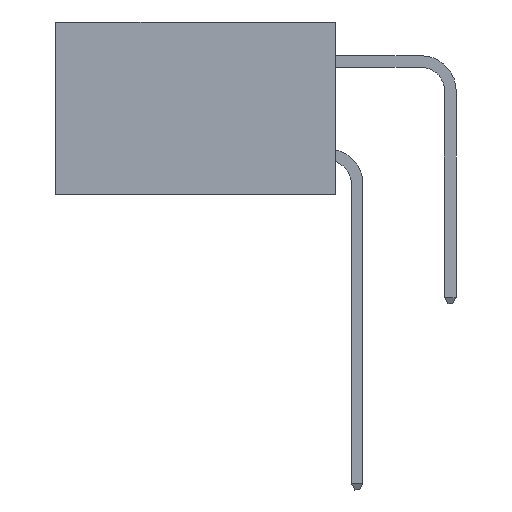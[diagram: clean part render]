
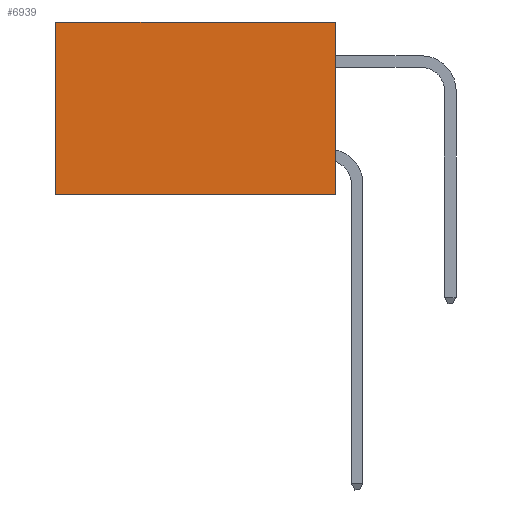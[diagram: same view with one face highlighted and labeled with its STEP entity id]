
A CAD part, left-side view. The second image highlights one B-rep face of the part: STEP entity #6939.
In plain terms, the highlighted planar face has unit normal (-1, 0, 0).
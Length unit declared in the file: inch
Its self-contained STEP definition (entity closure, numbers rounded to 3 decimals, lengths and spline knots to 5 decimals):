
#142 = CARTESIAN_POINT ( 'NONE',  ( 0.2875, 0.6, -0.37 ) ) ;
#578 = CARTESIAN_POINT ( 'NONE',  ( 0.2875, 0., -0.37 ) ) ;
#702 = CARTESIAN_POINT ( 'NONE',  ( 0.2875, 0., 0. ) ) ;
#854 = EDGE_CURVE ( 'NONE', #2070, #1374, #1759, .T. ) ;
#917 = LINE ( 'NONE', #3021, #9182 ) ;
#927 = CARTESIAN_POINT ( 'NONE',  ( 0.2875, 0.6, 0. ) ) ;
#1374 = VERTEX_POINT ( 'NONE', #142 ) ;
#1759 = LINE ( 'NONE', #578, #9862 ) ;
#1802 = DIRECTION ( 'NONE',  ( 0., 0., -1. ) ) ;
#2035 = AXIS2_PLACEMENT_3D ( 'NONE', #702, #8755, #4003 ) ;
#2070 = VERTEX_POINT ( 'NONE', #10262 ) ;
#2355 = VERTEX_POINT ( 'NONE', #4078 ) ;
#3021 = CARTESIAN_POINT ( 'NONE',  ( 0.2875, 0., 0. ) ) ;
#3191 = PLANE ( 'NONE',  #2035 ) ;
#3988 = VECTOR ( 'NONE', #9261, 39.37008 ) ;
#4003 = DIRECTION ( 'NONE',  ( 0., 0., -1. ) ) ;
#4078 = CARTESIAN_POINT ( 'NONE',  ( 0.2875, 0.6, 0. ) ) ;
#4181 = ORIENTED_EDGE ( 'NONE', *, *, #7413, .F. ) ;
#4833 = DIRECTION ( 'NONE',  ( 0., 1., 0. ) ) ;
#5002 = CARTESIAN_POINT ( 'NONE',  ( 0.2875, 0., 0. ) ) ;
#5904 = ORIENTED_EDGE ( 'NONE', *, *, #854, .F. ) ;
#6418 = LINE ( 'NONE', #927, #10190 ) ;
#6447 = EDGE_CURVE ( 'NONE', #2355, #1374, #6418, .T. ) ;
#6832 = EDGE_CURVE ( 'NONE', #7078, #2355, #917, .T. ) ;
#6939 = ADVANCED_FACE ( 'NONE', ( #8247 ), #3191, .F. ) ;
#7078 = VERTEX_POINT ( 'NONE', #5002 ) ;
#7413 = EDGE_CURVE ( 'NONE', #7078, #2070, #10174, .T. ) ;
#7451 = ORIENTED_EDGE ( 'NONE', *, *, #6832, .T. ) ;
#7495 = EDGE_LOOP ( 'NONE', ( #8118, #5904, #4181, #7451 ) ) ;
#7855 = DIRECTION ( 'NONE',  ( 0., 1., 0. ) ) ;
#8118 = ORIENTED_EDGE ( 'NONE', *, *, #6447, .T. ) ;
#8247 = FACE_OUTER_BOUND ( 'NONE', #7495, .T. ) ;
#8755 = DIRECTION ( 'NONE',  ( 1., 0., 0. ) ) ;
#9182 = VECTOR ( 'NONE', #7855, 39.37008 ) ;
#9261 = DIRECTION ( 'NONE',  ( 0., 0., -1. ) ) ;
#9862 = VECTOR ( 'NONE', #4833, 39.37008 ) ;
#9979 = CARTESIAN_POINT ( 'NONE',  ( 0.2875, 0., 0. ) ) ;
#10174 = LINE ( 'NONE', #9979, #3988 ) ;
#10190 = VECTOR ( 'NONE', #1802, 39.37008 ) ;
#10262 = CARTESIAN_POINT ( 'NONE',  ( 0.2875, 0., -0.37 ) ) ;
